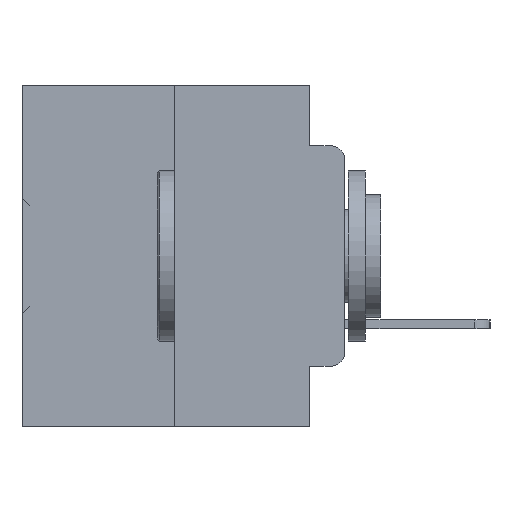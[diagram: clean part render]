
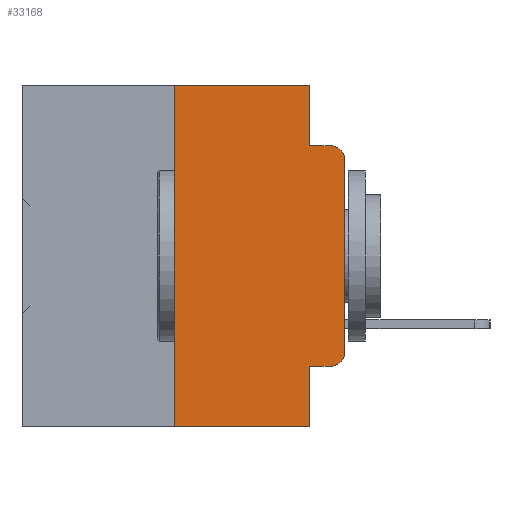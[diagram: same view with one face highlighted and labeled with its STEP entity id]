
A CAD part, left-side view. The second image highlights one B-rep face of the part: STEP entity #33168.
In plain terms, the highlighted planar face has unit normal (-1, 0, 0).
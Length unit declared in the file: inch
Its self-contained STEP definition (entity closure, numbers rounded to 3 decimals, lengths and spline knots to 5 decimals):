
#1757 = EDGE_CURVE ( 'NONE', #22874, #7299, #29502, .T. ) ;
#1893 = EDGE_LOOP ( 'NONE', ( #35315, #14520, #28900, #15004, #30774, #24810, #15480, #25263, #2554, #20173 ) ) ;
#2352 = CARTESIAN_POINT ( 'NONE',  ( 0., 0.473, 0. ) ) ;
#2484 = FACE_OUTER_BOUND ( 'NONE', #1893, .T. ) ;
#2554 = ORIENTED_EDGE ( 'NONE', *, *, #26078, .T. ) ;
#2631 = DIRECTION ( 'NONE',  ( 0., 0., 1. ) ) ;
#2675 = CARTESIAN_POINT ( 'NONE',  ( 0., 0.051, -0.0885 ) ) ;
#2896 = EDGE_CURVE ( 'NONE', #7299, #25807, #20180, .T. ) ;
#3941 = VECTOR ( 'NONE', #2631, 39.37008 ) ;
#4127 = VERTEX_POINT ( 'NONE', #11181 ) ;
#4181 = VERTEX_POINT ( 'NONE', #2675 ) ;
#4839 = PLANE ( 'NONE',  #15896 ) ;
#5310 = EDGE_CURVE ( 'NONE', #4181, #8764, #37748, .T. ) ;
#5366 = VECTOR ( 'NONE', #28454, 39.37008 ) ;
#5872 = DIRECTION ( 'NONE',  ( 0., -1., 0. ) ) ;
#7299 = VERTEX_POINT ( 'NONE', #26598 ) ;
#7504 = LINE ( 'NONE', #2352, #38026 ) ;
#8249 = DIRECTION ( 'NONE',  ( 0., -1., 0. ) ) ;
#8764 = VERTEX_POINT ( 'NONE', #18476 ) ;
#8920 = VECTOR ( 'NONE', #16847, 39.37008 ) ;
#10113 = DIRECTION ( 'NONE',  ( 0., 0., -1. ) ) ;
#11033 = AXIS2_PLACEMENT_3D ( 'NONE', #33333, #32497, #10113 ) ;
#11181 = CARTESIAN_POINT ( 'NONE',  ( 0., 0.051, -0.4115 ) ) ;
#11183 = DIRECTION ( 'NONE',  ( 0., 0., 1. ) ) ;
#11189 = EDGE_CURVE ( 'NONE', #4127, #34776, #31659, .T. ) ;
#11836 = EDGE_CURVE ( 'NONE', #33345, #32670, #7504, .T. ) ;
#12063 = CIRCLE ( 'NONE', #17790, 0.02 ) ;
#13668 = CARTESIAN_POINT ( 'NONE',  ( 0., 0.051, -0.0885 ) ) ;
#13752 = DIRECTION ( 'NONE',  ( 1., 0., 0. ) ) ;
#14520 = ORIENTED_EDGE ( 'NONE', *, *, #21021, .T. ) ;
#15004 = ORIENTED_EDGE ( 'NONE', *, *, #33298, .F. ) ;
#15230 = LINE ( 'NONE', #26618, #37864 ) ;
#15480 = ORIENTED_EDGE ( 'NONE', *, *, #28778, .T. ) ;
#15896 = AXIS2_PLACEMENT_3D ( 'NONE', #31533, #13752, #34448 ) ;
#16368 = CARTESIAN_POINT ( 'NONE',  ( 0., 0.473, -0.5 ) ) ;
#16730 = DIRECTION ( 'NONE',  ( -1., 0., 0. ) ) ;
#16847 = DIRECTION ( 'NONE',  ( 0., 0., -1. ) ) ;
#17790 = AXIS2_PLACEMENT_3D ( 'NONE', #34422, #16730, #37378 ) ;
#17917 = CARTESIAN_POINT ( 'NONE',  ( 0., 0.051, -0.5 ) ) ;
#18476 = CARTESIAN_POINT ( 'NONE',  ( 0., 0.02, -0.0885 ) ) ;
#19709 = LINE ( 'NONE', #38015, #3941 ) ;
#20173 = ORIENTED_EDGE ( 'NONE', *, *, #1757, .T. ) ;
#20180 = LINE ( 'NONE', #30339, #34912 ) ;
#20420 = DIRECTION ( 'NONE',  ( 0., 0., -1. ) ) ;
#20500 = CARTESIAN_POINT ( 'NONE',  ( 0., 0.25, -0.5 ) ) ;
#21021 = EDGE_CURVE ( 'NONE', #25807, #8764, #12063, .T. ) ;
#21490 = LINE ( 'NONE', #35083, #28379 ) ;
#22364 = LINE ( 'NONE', #16368, #37971 ) ;
#22874 = VERTEX_POINT ( 'NONE', #37118 ) ;
#24810 = ORIENTED_EDGE ( 'NONE', *, *, #32088, .F. ) ;
#25263 = ORIENTED_EDGE ( 'NONE', *, *, #11189, .F. ) ;
#25807 = VERTEX_POINT ( 'NONE', #37176 ) ;
#26078 = EDGE_CURVE ( 'NONE', #4127, #22874, #15230, .T. ) ;
#26598 = CARTESIAN_POINT ( 'NONE',  ( 0., 0., -0.3915 ) ) ;
#26618 = CARTESIAN_POINT ( 'NONE',  ( 0., 0.051, -0.4115 ) ) ;
#27715 = VERTEX_POINT ( 'NONE', #20500 ) ;
#28379 = VECTOR ( 'NONE', #20420, 39.37008 ) ;
#28454 = DIRECTION ( 'NONE',  ( 0., -1., 0. ) ) ;
#28778 = EDGE_CURVE ( 'NONE', #27715, #34776, #22364, .T. ) ;
#28900 = ORIENTED_EDGE ( 'NONE', *, *, #5310, .F. ) ;
#29502 = CIRCLE ( 'NONE', #11033, 0.02 ) ;
#30339 = CARTESIAN_POINT ( 'NONE',  ( 0., 0., 0. ) ) ;
#30774 = ORIENTED_EDGE ( 'NONE', *, *, #11836, .F. ) ;
#31533 = CARTESIAN_POINT ( 'NONE',  ( 0., 0.473, 0. ) ) ;
#31659 = LINE ( 'NONE', #37511, #8920 ) ;
#31822 = CARTESIAN_POINT ( 'NONE',  ( 0., 0.051, 0. ) ) ;
#32088 = EDGE_CURVE ( 'NONE', #27715, #33345, #19709, .T. ) ;
#32276 = CARTESIAN_POINT ( 'NONE',  ( 0., 0.25, 0. ) ) ;
#32497 = DIRECTION ( 'NONE',  ( -1., 0., 0. ) ) ;
#32670 = VERTEX_POINT ( 'NONE', #31822 ) ;
#33168 = ADVANCED_FACE ( 'NONE', ( #2484 ), #4839, .F. ) ;
#33298 = EDGE_CURVE ( 'NONE', #32670, #4181, #21490, .T. ) ;
#33333 = CARTESIAN_POINT ( 'NONE',  ( 0., 0.02, -0.3915 ) ) ;
#33345 = VERTEX_POINT ( 'NONE', #32276 ) ;
#34422 = CARTESIAN_POINT ( 'NONE',  ( 0., 0.02, -0.1085 ) ) ;
#34448 = DIRECTION ( 'NONE',  ( 0., 0., -1. ) ) ;
#34776 = VERTEX_POINT ( 'NONE', #17917 ) ;
#34912 = VECTOR ( 'NONE', #11183, 39.37008 ) ;
#35083 = CARTESIAN_POINT ( 'NONE',  ( 0., 0.051, 0. ) ) ;
#35315 = ORIENTED_EDGE ( 'NONE', *, *, #2896, .T. ) ;
#37036 = DIRECTION ( 'NONE',  ( 0., -1., 0. ) ) ;
#37118 = CARTESIAN_POINT ( 'NONE',  ( 0., 0.02, -0.4115 ) ) ;
#37176 = CARTESIAN_POINT ( 'NONE',  ( 0., 0., -0.1085 ) ) ;
#37378 = DIRECTION ( 'NONE',  ( 0., 0., -1. ) ) ;
#37511 = CARTESIAN_POINT ( 'NONE',  ( 0., 0.051, 0. ) ) ;
#37748 = LINE ( 'NONE', #13668, #5366 ) ;
#37864 = VECTOR ( 'NONE', #5872, 39.37008 ) ;
#37971 = VECTOR ( 'NONE', #37036, 39.37008 ) ;
#38015 = CARTESIAN_POINT ( 'NONE',  ( 0., 0.25, 0. ) ) ;
#38026 = VECTOR ( 'NONE', #8249, 39.37008 ) ;
